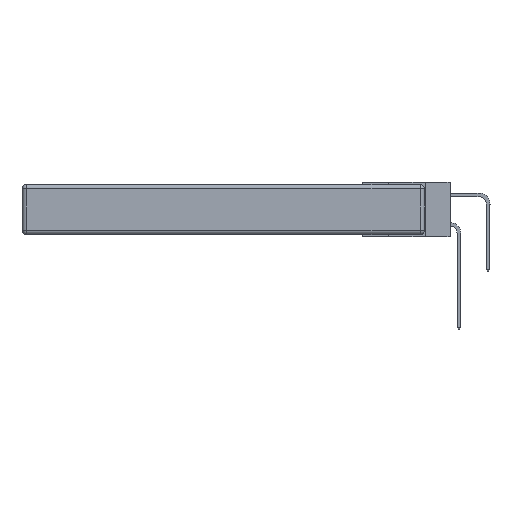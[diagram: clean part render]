
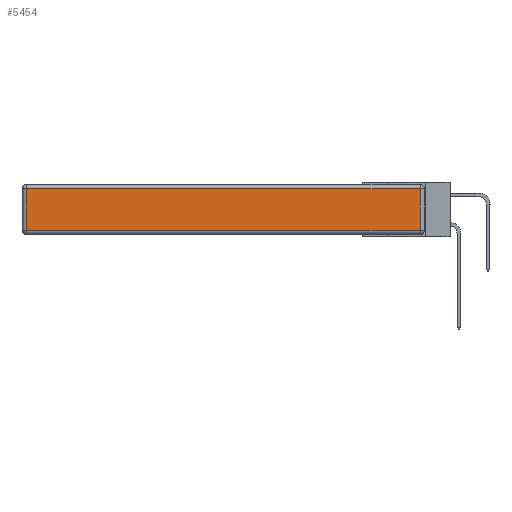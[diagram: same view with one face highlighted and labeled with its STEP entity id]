
A CAD part, left-side view. The second image highlights one B-rep face of the part: STEP entity #5454.
In plain terms, the highlighted planar face has unit normal (-1, 0, 0).
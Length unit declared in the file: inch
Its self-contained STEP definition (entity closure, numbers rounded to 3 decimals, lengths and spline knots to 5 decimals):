
#456 = VERTEX_POINT ( 'NONE', #14006 ) ;
#479 = LINE ( 'NONE', #9606, #14266 ) ;
#2283 = VERTEX_POINT ( 'NONE', #15825 ) ;
#2726 = DIRECTION ( 'NONE',  ( 0., 1., 0. ) ) ;
#4455 = LINE ( 'NONE', #7350, #9450 ) ;
#4832 = ORIENTED_EDGE ( 'NONE', *, *, #15658, .T. ) ;
#5018 = DIRECTION ( 'NONE',  ( -1., 0., 0. ) ) ;
#5045 = VERTEX_POINT ( 'NONE', #10109 ) ;
#5373 = CARTESIAN_POINT ( 'NONE',  ( 0., 2.75, -0.03 ) ) ;
#5379 = DIRECTION ( 'NONE',  ( 0., 0., 1. ) ) ;
#5454 = ADVANCED_FACE ( 'NONE', ( #13958 ), #14293, .T. ) ;
#5865 = ORIENTED_EDGE ( 'NONE', *, *, #9072, .T. ) ;
#6229 = ORIENTED_EDGE ( 'NONE', *, *, #15446, .T. ) ;
#6518 = AXIS2_PLACEMENT_3D ( 'NONE', #7735, #5018, #8972 ) ;
#7350 = CARTESIAN_POINT ( 'NONE',  ( 0., 2.72, -0.343 ) ) ;
#7735 = CARTESIAN_POINT ( 'NONE',  ( 0., 0., -0.343 ) ) ;
#8254 = DIRECTION ( 'NONE',  ( 0., -1., 0. ) ) ;
#8972 = DIRECTION ( 'NONE',  ( 0., 0., 1. ) ) ;
#9072 = EDGE_CURVE ( 'NONE', #16035, #2283, #15501, .T. ) ;
#9450 = VECTOR ( 'NONE', #15346, 39.37008 ) ;
#9606 = CARTESIAN_POINT ( 'NONE',  ( 0., 0., -0.313 ) ) ;
#10109 = CARTESIAN_POINT ( 'NONE',  ( 0., 2.72, -0.03 ) ) ;
#11494 = ORIENTED_EDGE ( 'NONE', *, *, #15950, .T. ) ;
#12172 = EDGE_LOOP ( 'NONE', ( #11494, #5865, #6229, #4832 ) ) ;
#12357 = VECTOR ( 'NONE', #5379, 39.37008 ) ;
#13332 = VECTOR ( 'NONE', #2726, 39.37008 ) ;
#13645 = CARTESIAN_POINT ( 'NONE',  ( 0., 0.03, -0.313 ) ) ;
#13958 = FACE_OUTER_BOUND ( 'NONE', #12172, .T. ) ;
#14006 = CARTESIAN_POINT ( 'NONE',  ( 0., 2.72, -0.313 ) ) ;
#14266 = VECTOR ( 'NONE', #8254, 39.37008 ) ;
#14293 = PLANE ( 'NONE',  #6518 ) ;
#15346 = DIRECTION ( 'NONE',  ( 0., 0., -1. ) ) ;
#15446 = EDGE_CURVE ( 'NONE', #2283, #5045, #16053, .T. ) ;
#15501 = LINE ( 'NONE', #16284, #12357 ) ;
#15658 = EDGE_CURVE ( 'NONE', #5045, #456, #4455, .T. ) ;
#15825 = CARTESIAN_POINT ( 'NONE',  ( 0., 0.03, -0.03 ) ) ;
#15950 = EDGE_CURVE ( 'NONE', #456, #16035, #479, .T. ) ;
#16035 = VERTEX_POINT ( 'NONE', #13645 ) ;
#16053 = LINE ( 'NONE', #5373, #13332 ) ;
#16284 = CARTESIAN_POINT ( 'NONE',  ( 0., 0.03, -0.343 ) ) ;
